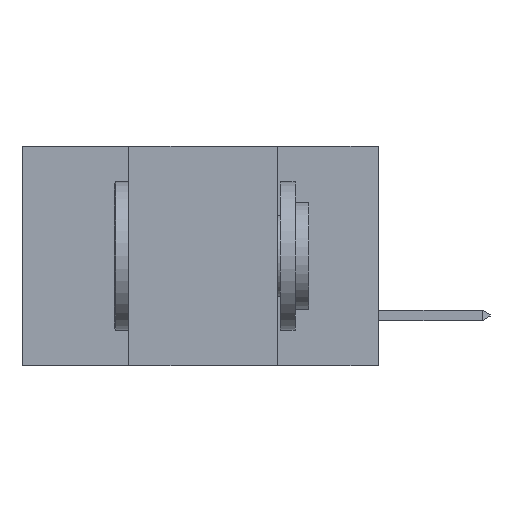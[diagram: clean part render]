
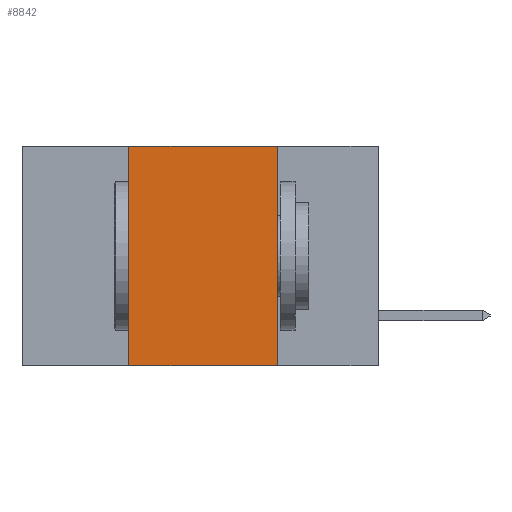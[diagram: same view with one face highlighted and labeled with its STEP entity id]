
A CAD part, left-side view. The second image highlights one B-rep face of the part: STEP entity #8842.
In plain terms, the highlighted planar face has unit normal (-1, 0, 0).
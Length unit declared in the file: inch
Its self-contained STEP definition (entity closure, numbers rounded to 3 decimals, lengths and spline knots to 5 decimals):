
#432 = VERTEX_POINT ( 'NONE', #4431 ) ;
#683 = LINE ( 'NONE', #2825, #13840 ) ;
#1186 = CARTESIAN_POINT ( 'NONE',  ( 0., 0.42, -0.37 ) ) ;
#1530 = VECTOR ( 'NONE', #17409, 39.37008 ) ;
#1787 = LINE ( 'NONE', #8736, #15481 ) ;
#2561 = EDGE_CURVE ( 'NONE', #13235, #18593, #1787, .T. ) ;
#2777 = EDGE_CURVE ( 'NONE', #8371, #432, #10677, .T. ) ;
#2825 = CARTESIAN_POINT ( 'NONE',  ( 0., 0.6, -0.37 ) ) ;
#3241 = ORIENTED_EDGE ( 'NONE', *, *, #2561, .F. ) ;
#3652 = DIRECTION ( 'NONE',  ( 0., -1., 0. ) ) ;
#3938 = EDGE_CURVE ( 'NONE', #8371, #18593, #683, .T. ) ;
#4309 = DIRECTION ( 'NONE',  ( 1., 0., 0. ) ) ;
#4338 = DIRECTION ( 'NONE',  ( 0., 0., -1. ) ) ;
#4384 = CARTESIAN_POINT ( 'NONE',  ( 0., 0.6, 0. ) ) ;
#4431 = CARTESIAN_POINT ( 'NONE',  ( 0., 0.42, 0. ) ) ;
#4455 = PLANE ( 'NONE',  #15043 ) ;
#4672 = ORIENTED_EDGE ( 'NONE', *, *, #2777, .F. ) ;
#6615 = VECTOR ( 'NONE', #16304, 39.37008 ) ;
#7787 = ORIENTED_EDGE ( 'NONE', *, *, #3938, .T. ) ;
#8371 = VERTEX_POINT ( 'NONE', #1186 ) ;
#8578 = EDGE_CURVE ( 'NONE', #432, #13235, #15178, .T. ) ;
#8736 = CARTESIAN_POINT ( 'NONE',  ( 0., 0.17, -0.37 ) ) ;
#8811 = DIRECTION ( 'NONE',  ( 0., 0., -1. ) ) ;
#8842 = ADVANCED_FACE ( 'NONE', ( #14383 ), #4455, .F. ) ;
#10404 = CARTESIAN_POINT ( 'NONE',  ( 0., 0.17, 0. ) ) ;
#10677 = LINE ( 'NONE', #17215, #1530 ) ;
#13235 = VERTEX_POINT ( 'NONE', #10404 ) ;
#13840 = VECTOR ( 'NONE', #3652, 39.37008 ) ;
#14383 = FACE_OUTER_BOUND ( 'NONE', #18764, .T. ) ;
#14616 = CARTESIAN_POINT ( 'NONE',  ( 0., 0.17, -0.37 ) ) ;
#15043 = AXIS2_PLACEMENT_3D ( 'NONE', #4384, #4309, #4338 ) ;
#15090 = ORIENTED_EDGE ( 'NONE', *, *, #8578, .F. ) ;
#15178 = LINE ( 'NONE', #15695, #6615 ) ;
#15481 = VECTOR ( 'NONE', #8811, 39.37008 ) ;
#15695 = CARTESIAN_POINT ( 'NONE',  ( 0., 0.6, 0. ) ) ;
#16304 = DIRECTION ( 'NONE',  ( 0., -1., 0. ) ) ;
#17215 = CARTESIAN_POINT ( 'NONE',  ( 0., 0.42, -0.37 ) ) ;
#17409 = DIRECTION ( 'NONE',  ( 0., 0., 1. ) ) ;
#18593 = VERTEX_POINT ( 'NONE', #14616 ) ;
#18764 = EDGE_LOOP ( 'NONE', ( #3241, #15090, #4672, #7787 ) ) ;
